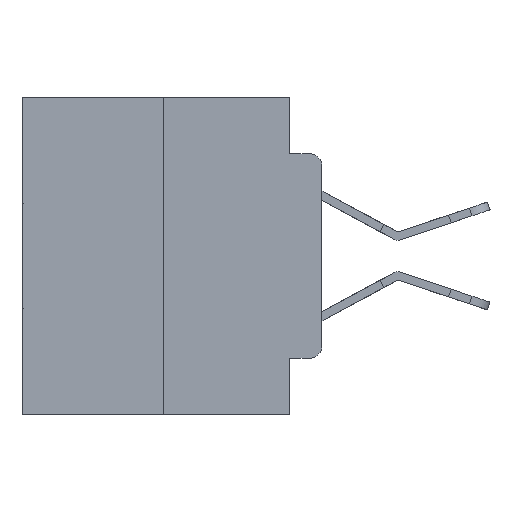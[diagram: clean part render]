
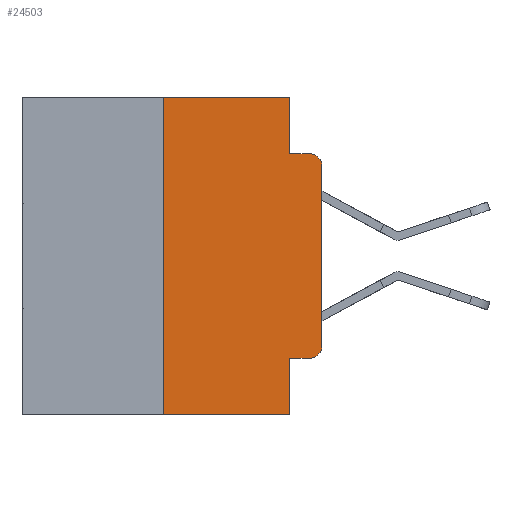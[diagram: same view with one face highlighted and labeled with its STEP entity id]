
A CAD part, left-side view. The second image highlights one B-rep face of the part: STEP entity #24503.
In plain terms, the highlighted planar face has unit normal (-1, 0, 0).
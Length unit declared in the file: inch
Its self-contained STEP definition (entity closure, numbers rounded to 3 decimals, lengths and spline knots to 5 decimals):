
#479 = CIRCLE ( 'NONE', #25098, 0.02 ) ;
#2369 = LINE ( 'NONE', #13227, #24585 ) ;
#2547 = LINE ( 'NONE', #7325, #13925 ) ;
#2617 = CARTESIAN_POINT ( 'NONE',  ( 0., 0.051, -0.0885 ) ) ;
#2740 = EDGE_CURVE ( 'NONE', #12015, #11329, #9273, .T. ) ;
#3108 = AXIS2_PLACEMENT_3D ( 'NONE', #19905, #6643, #22073 ) ;
#3141 = VERTEX_POINT ( 'NONE', #20522 ) ;
#3460 = VECTOR ( 'NONE', #26677, 39.37008 ) ;
#3516 = CARTESIAN_POINT ( 'NONE',  ( 0., 0.25, 0. ) ) ;
#4104 = DIRECTION ( 'NONE',  ( 0., 0., 1. ) ) ;
#4345 = PLANE ( 'NONE',  #3108 ) ;
#5390 = CARTESIAN_POINT ( 'NONE',  ( 0., 0.25, -0.5 ) ) ;
#5921 = DIRECTION ( 'NONE',  ( -1., 0., 0. ) ) ;
#5933 = EDGE_CURVE ( 'NONE', #11329, #11067, #6316, .T. ) ;
#6316 = LINE ( 'NONE', #15820, #11601 ) ;
#6334 = VECTOR ( 'NONE', #9923, 39.37008 ) ;
#6643 = DIRECTION ( 'NONE',  ( 1., 0., 0. ) ) ;
#6668 = CARTESIAN_POINT ( 'NONE',  ( 0., 0.02, -0.1085 ) ) ;
#6776 = DIRECTION ( 'NONE',  ( 0., 0., 1. ) ) ;
#7325 = CARTESIAN_POINT ( 'NONE',  ( 0., 0.051, -0.4115 ) ) ;
#7604 = CARTESIAN_POINT ( 'NONE',  ( 0., 0.051, -0.0885 ) ) ;
#8987 = DIRECTION ( 'NONE',  ( 0., 0., -1. ) ) ;
#9229 = VERTEX_POINT ( 'NONE', #3516 ) ;
#9273 = CIRCLE ( 'NONE', #16130, 0.02 ) ;
#9923 = DIRECTION ( 'NONE',  ( 0., 0., -1. ) ) ;
#10402 = VECTOR ( 'NONE', #4104, 39.37008 ) ;
#10527 = VERTEX_POINT ( 'NONE', #28001 ) ;
#10632 = EDGE_CURVE ( 'NONE', #9229, #3141, #2369, .T. ) ;
#10746 = ORIENTED_EDGE ( 'NONE', *, *, #10632, .F. ) ;
#10785 = EDGE_CURVE ( 'NONE', #3141, #22428, #21241, .T. ) ;
#10920 = VERTEX_POINT ( 'NONE', #20708 ) ;
#10978 = DIRECTION ( 'NONE',  ( 0., -1., 0. ) ) ;
#11067 = VERTEX_POINT ( 'NONE', #14751 ) ;
#11329 = VERTEX_POINT ( 'NONE', #24155 ) ;
#11331 = EDGE_CURVE ( 'NONE', #11067, #25571, #479, .T. ) ;
#11463 = CARTESIAN_POINT ( 'NONE',  ( 0., 0.02, -0.4115 ) ) ;
#11539 = CARTESIAN_POINT ( 'NONE',  ( 0., 0.051, 0. ) ) ;
#11601 = VECTOR ( 'NONE', #6776, 39.37008 ) ;
#12015 = VERTEX_POINT ( 'NONE', #11463 ) ;
#12310 = LINE ( 'NONE', #27272, #6334 ) ;
#12531 = EDGE_CURVE ( 'NONE', #13761, #10920, #22193, .T. ) ;
#13227 = CARTESIAN_POINT ( 'NONE',  ( 0., 0.473, 0. ) ) ;
#13761 = VERTEX_POINT ( 'NONE', #5390 ) ;
#13925 = VECTOR ( 'NONE', #26997, 39.37008 ) ;
#14193 = VECTOR ( 'NONE', #26933, 39.37008 ) ;
#14751 = CARTESIAN_POINT ( 'NONE',  ( 0., 0., -0.1085 ) ) ;
#14921 = LINE ( 'NONE', #2617, #14193 ) ;
#14972 = ORIENTED_EDGE ( 'NONE', *, *, #18335, .T. ) ;
#15277 = EDGE_CURVE ( 'NONE', #13761, #9229, #21368, .T. ) ;
#15820 = CARTESIAN_POINT ( 'NONE',  ( 0., 0., 0. ) ) ;
#15823 = EDGE_CURVE ( 'NONE', #22428, #25571, #14921, .T. ) ;
#16130 = AXIS2_PLACEMENT_3D ( 'NONE', #19223, #5921, #21394 ) ;
#17331 = ORIENTED_EDGE ( 'NONE', *, *, #21948, .F. ) ;
#18335 = EDGE_CURVE ( 'NONE', #10527, #12015, #2547, .T. ) ;
#18784 = EDGE_LOOP ( 'NONE', ( #22988, #19973, #21337, #25350, #10746, #25023, #21710, #17331, #14972, #24089 ) ) ;
#19223 = CARTESIAN_POINT ( 'NONE',  ( 0., 0.02, -0.3915 ) ) ;
#19687 = CARTESIAN_POINT ( 'NONE',  ( 0., 0.25, 0. ) ) ;
#19905 = CARTESIAN_POINT ( 'NONE',  ( 0., 0.473, 0. ) ) ;
#19973 = ORIENTED_EDGE ( 'NONE', *, *, #11331, .T. ) ;
#20522 = CARTESIAN_POINT ( 'NONE',  ( 0., 0.051, 0. ) ) ;
#20708 = CARTESIAN_POINT ( 'NONE',  ( 0., 0.051, -0.5 ) ) ;
#20866 = CARTESIAN_POINT ( 'NONE',  ( 0., 0.473, -0.5 ) ) ;
#21241 = LINE ( 'NONE', #11539, #3460 ) ;
#21337 = ORIENTED_EDGE ( 'NONE', *, *, #15823, .F. ) ;
#21368 = LINE ( 'NONE', #19687, #10402 ) ;
#21394 = DIRECTION ( 'NONE',  ( 0., 0., -1. ) ) ;
#21710 = ORIENTED_EDGE ( 'NONE', *, *, #12531, .T. ) ;
#21861 = CARTESIAN_POINT ( 'NONE',  ( 0., 0.02, -0.0885 ) ) ;
#21948 = EDGE_CURVE ( 'NONE', #10527, #10920, #12310, .T. ) ;
#22073 = DIRECTION ( 'NONE',  ( 0., 0., -1. ) ) ;
#22101 = DIRECTION ( 'NONE',  ( -1., 0., 0. ) ) ;
#22193 = LINE ( 'NONE', #20866, #25865 ) ;
#22428 = VERTEX_POINT ( 'NONE', #7604 ) ;
#22988 = ORIENTED_EDGE ( 'NONE', *, *, #5933, .T. ) ;
#23007 = DIRECTION ( 'NONE',  ( 0., -1., 0. ) ) ;
#24089 = ORIENTED_EDGE ( 'NONE', *, *, #2740, .T. ) ;
#24155 = CARTESIAN_POINT ( 'NONE',  ( 0., 0., -0.3915 ) ) ;
#24344 = FACE_OUTER_BOUND ( 'NONE', #18784, .T. ) ;
#24503 = ADVANCED_FACE ( 'NONE', ( #24344 ), #4345, .F. ) ;
#24585 = VECTOR ( 'NONE', #10978, 39.37008 ) ;
#25023 = ORIENTED_EDGE ( 'NONE', *, *, #15277, .F. ) ;
#25098 = AXIS2_PLACEMENT_3D ( 'NONE', #6668, #22101, #8987 ) ;
#25350 = ORIENTED_EDGE ( 'NONE', *, *, #10785, .F. ) ;
#25571 = VERTEX_POINT ( 'NONE', #21861 ) ;
#25865 = VECTOR ( 'NONE', #23007, 39.37008 ) ;
#26677 = DIRECTION ( 'NONE',  ( 0., 0., -1. ) ) ;
#26933 = DIRECTION ( 'NONE',  ( 0., -1., 0. ) ) ;
#26997 = DIRECTION ( 'NONE',  ( 0., -1., 0. ) ) ;
#27272 = CARTESIAN_POINT ( 'NONE',  ( 0., 0.051, 0. ) ) ;
#28001 = CARTESIAN_POINT ( 'NONE',  ( 0., 0.051, -0.4115 ) ) ;
